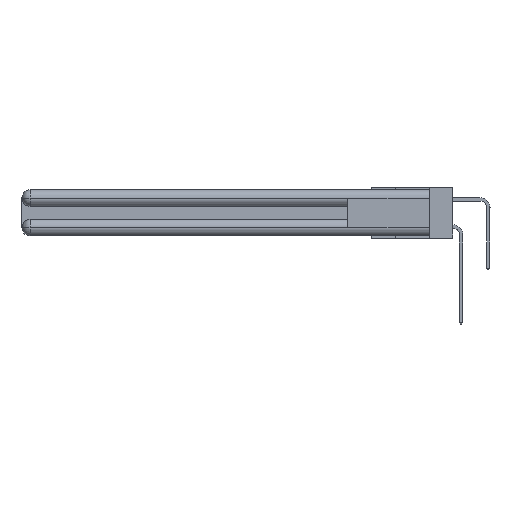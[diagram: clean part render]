
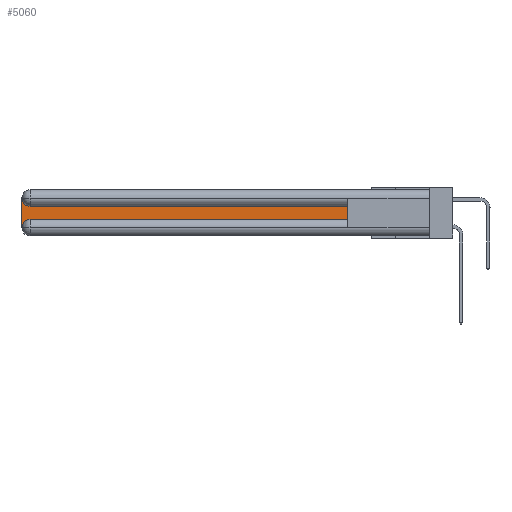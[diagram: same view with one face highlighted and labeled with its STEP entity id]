
A CAD part, left-side view. The second image highlights one B-rep face of the part: STEP entity #5060.
In plain terms, the highlighted planar face has unit normal (-1, 0, 0).
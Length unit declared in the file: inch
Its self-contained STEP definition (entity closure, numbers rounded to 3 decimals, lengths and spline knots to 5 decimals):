
#78 = CIRCLE ( 'NONE', #2600, 0.06 ) ;
#340 = LINE ( 'NONE', #6824, #29082 ) ;
#955 = CARTESIAN_POINT ( 'NONE',  ( 0.075, 3., -0.2775 ) ) ;
#1095 = DIRECTION ( 'NONE',  ( 0., -1., 0. ) ) ;
#1367 = EDGE_LOOP ( 'NONE', ( #30578, #4990, #16463, #15056, #16429, #8422 ) ) ;
#1842 = VERTEX_POINT ( 'NONE', #21913 ) ;
#2580 = EDGE_CURVE ( 'NONE', #16057, #1842, #340, .T. ) ;
#2600 = AXIS2_PLACEMENT_3D ( 'NONE', #25832, #31451, #37225 ) ;
#3885 = EDGE_CURVE ( 'NONE', #29029, #11983, #15114, .T. ) ;
#4413 = CARTESIAN_POINT ( 'NONE',  ( 0.075, 3., -0.1225 ) ) ;
#4545 = DIRECTION ( 'NONE',  ( 0., 0., -1. ) ) ;
#4990 = ORIENTED_EDGE ( 'NONE', *, *, #22751, .T. ) ;
#5060 = ADVANCED_FACE ( 'NONE', ( #9648 ), #13613, .F. ) ;
#6704 = AXIS2_PLACEMENT_3D ( 'NONE', #4413, #16510, #4545 ) ;
#6824 = CARTESIAN_POINT ( 'NONE',  ( 0.075, 0.6, -0.2175 ) ) ;
#7142 = CARTESIAN_POINT ( 'NONE',  ( 0.075, 0.6, -0.1225 ) ) ;
#8422 = ORIENTED_EDGE ( 'NONE', *, *, #24565, .T. ) ;
#9388 = CARTESIAN_POINT ( 'NONE',  ( 0.075, 3., -0.2175 ) ) ;
#9648 = FACE_OUTER_BOUND ( 'NONE', #1367, .T. ) ;
#9726 = CIRCLE ( 'NONE', #36734, 0.06 ) ;
#11983 = VERTEX_POINT ( 'NONE', #33815 ) ;
#13613 = PLANE ( 'NONE',  #6704 ) ;
#13622 = VECTOR ( 'NONE', #34179, 39.37008 ) ;
#15056 = ORIENTED_EDGE ( 'NONE', *, *, #18829, .T. ) ;
#15114 = LINE ( 'NONE', #19285, #26970 ) ;
#16057 = VERTEX_POINT ( 'NONE', #24434 ) ;
#16429 = ORIENTED_EDGE ( 'NONE', *, *, #2580, .T. ) ;
#16463 = ORIENTED_EDGE ( 'NONE', *, *, #23384, .T. ) ;
#16510 = DIRECTION ( 'NONE',  ( 1., 0., 0. ) ) ;
#17335 = LINE ( 'NONE', #9388, #34692 ) ;
#18781 = VERTEX_POINT ( 'NONE', #955 ) ;
#18829 = EDGE_CURVE ( 'NONE', #18781, #16057, #9726, .T. ) ;
#19285 = CARTESIAN_POINT ( 'NONE',  ( 0.075, 0.6, -0.1225 ) ) ;
#21146 = DIRECTION ( 'NONE',  ( 0., 0., -1. ) ) ;
#21913 = CARTESIAN_POINT ( 'NONE',  ( 0.075, 0.6, -0.2175 ) ) ;
#22202 = VERTEX_POINT ( 'NONE', #24885 ) ;
#22751 = EDGE_CURVE ( 'NONE', #11983, #22202, #78, .T. ) ;
#22948 = CARTESIAN_POINT ( 'NONE',  ( 0.075, 0.6, -0.2175 ) ) ;
#23384 = EDGE_CURVE ( 'NONE', #22202, #18781, #17335, .T. ) ;
#24434 = CARTESIAN_POINT ( 'NONE',  ( 0.075, 2.94, -0.2175 ) ) ;
#24565 = EDGE_CURVE ( 'NONE', #1842, #29029, #36899, .T. ) ;
#24885 = CARTESIAN_POINT ( 'NONE',  ( 0.075, 3., -0.0625 ) ) ;
#25775 = CARTESIAN_POINT ( 'NONE',  ( 0.075, 2.94, -0.2775 ) ) ;
#25832 = CARTESIAN_POINT ( 'NONE',  ( 0.075, 2.94, -0.0625 ) ) ;
#26970 = VECTOR ( 'NONE', #28948, 39.37008 ) ;
#28577 = DIRECTION ( 'NONE',  ( 1., 0., 0. ) ) ;
#28948 = DIRECTION ( 'NONE',  ( 0., 1., 0. ) ) ;
#29029 = VERTEX_POINT ( 'NONE', #7142 ) ;
#29082 = VECTOR ( 'NONE', #1095, 39.37008 ) ;
#30578 = ORIENTED_EDGE ( 'NONE', *, *, #3885, .T. ) ;
#31451 = DIRECTION ( 'NONE',  ( 1., 0., 0. ) ) ;
#31521 = DIRECTION ( 'NONE',  ( 0., 0., -1. ) ) ;
#33815 = CARTESIAN_POINT ( 'NONE',  ( 0.075, 2.94, -0.1225 ) ) ;
#34179 = DIRECTION ( 'NONE',  ( 0., 0., 1. ) ) ;
#34692 = VECTOR ( 'NONE', #21146, 39.37008 ) ;
#36734 = AXIS2_PLACEMENT_3D ( 'NONE', #25775, #28577, #31521 ) ;
#36899 = LINE ( 'NONE', #22948, #13622 ) ;
#37225 = DIRECTION ( 'NONE',  ( 0., 0., -1. ) ) ;
